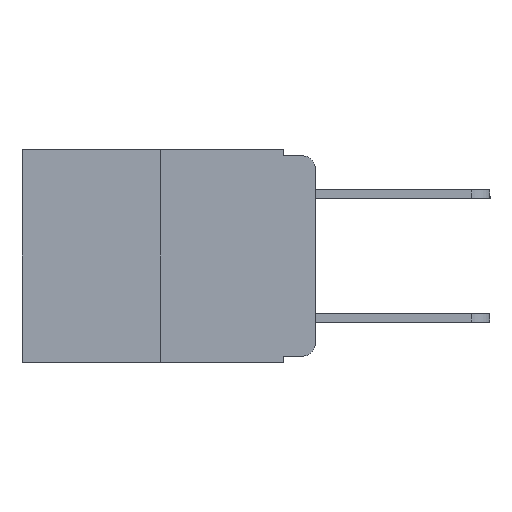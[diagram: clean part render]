
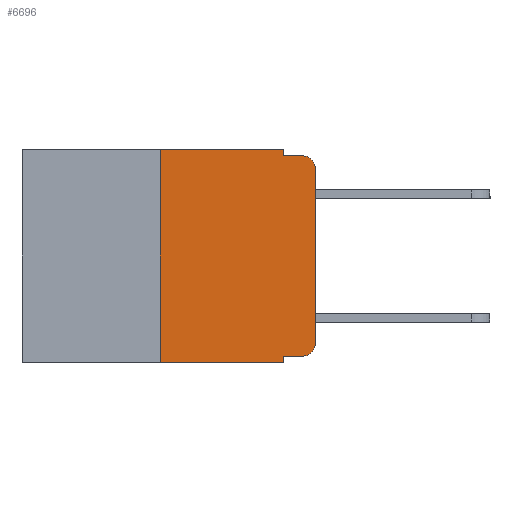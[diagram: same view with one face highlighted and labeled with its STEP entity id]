
A CAD part, left-side view. The second image highlights one B-rep face of the part: STEP entity #6696.
In plain terms, the highlighted planar face has unit normal (-1, 0, 0).
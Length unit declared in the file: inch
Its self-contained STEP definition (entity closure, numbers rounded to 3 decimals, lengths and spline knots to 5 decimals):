
#28 = LINE ( 'NONE', #1433, #3283 ) ;
#178 = CARTESIAN_POINT ( 'NONE',  ( 0., 0.051, -0.01 ) ) ;
#351 = DIRECTION ( 'NONE',  ( 0., 0., 1. ) ) ;
#733 = ORIENTED_EDGE ( 'NONE', *, *, #8186, .F. ) ;
#751 = ORIENTED_EDGE ( 'NONE', *, *, #13376, .T. ) ;
#1317 = VERTEX_POINT ( 'NONE', #10556 ) ;
#1433 = CARTESIAN_POINT ( 'NONE',  ( 0., 0.473, 0. ) ) ;
#1447 = DIRECTION ( 'NONE',  ( 0., -1., 0. ) ) ;
#2100 = ORIENTED_EDGE ( 'NONE', *, *, #13353, .T. ) ;
#2632 = DIRECTION ( 'NONE',  ( 0., -1., 0. ) ) ;
#3283 = VECTOR ( 'NONE', #2632, 39.37008 ) ;
#3311 = ORIENTED_EDGE ( 'NONE', *, *, #7199, .F. ) ;
#3335 = CARTESIAN_POINT ( 'NONE',  ( 0., 0.051, -0.333 ) ) ;
#3402 = ORIENTED_EDGE ( 'NONE', *, *, #8897, .T. ) ;
#3748 = FACE_OUTER_BOUND ( 'NONE', #5671, .T. ) ;
#3941 = VERTEX_POINT ( 'NONE', #10624 ) ;
#4159 = CARTESIAN_POINT ( 'NONE',  ( 0., 0., -0.313 ) ) ;
#4176 = DIRECTION ( 'NONE',  ( 0., 0., -1. ) ) ;
#4203 = LINE ( 'NONE', #178, #12463 ) ;
#4214 = CARTESIAN_POINT ( 'NONE',  ( 0., 0.25, 0. ) ) ;
#4242 = VECTOR ( 'NONE', #8245, 39.37008 ) ;
#4402 = VECTOR ( 'NONE', #13381, 39.37008 ) ;
#4470 = ORIENTED_EDGE ( 'NONE', *, *, #7860, .F. ) ;
#5124 = EDGE_CURVE ( 'NONE', #14193, #6923, #11903, .T. ) ;
#5505 = VERTEX_POINT ( 'NONE', #7129 ) ;
#5671 = EDGE_LOOP ( 'NONE', ( #13999, #6359, #7160, #733, #12368, #4470, #3402, #3311, #2100, #751 ) ) ;
#5741 = AXIS2_PLACEMENT_3D ( 'NONE', #7188, #6296, #4176 ) ;
#6055 = CARTESIAN_POINT ( 'NONE',  ( 0., 0.25, -0.343 ) ) ;
#6296 = DIRECTION ( 'NONE',  ( 1., 0., 0. ) ) ;
#6359 = ORIENTED_EDGE ( 'NONE', *, *, #5124, .T. ) ;
#6367 = CARTESIAN_POINT ( 'NONE',  ( 0., 0.051, 0. ) ) ;
#6696 = ADVANCED_FACE ( 'NONE', ( #3748 ), #10330, .F. ) ;
#6923 = VERTEX_POINT ( 'NONE', #14333 ) ;
#6975 = CARTESIAN_POINT ( 'NONE',  ( 0., 0.02, -0.313 ) ) ;
#7129 = CARTESIAN_POINT ( 'NONE',  ( 0., 0.051, -0.01 ) ) ;
#7160 = ORIENTED_EDGE ( 'NONE', *, *, #13539, .F. ) ;
#7188 = CARTESIAN_POINT ( 'NONE',  ( 0., 0.473, 0. ) ) ;
#7199 = EDGE_CURVE ( 'NONE', #3941, #11550, #14495, .T. ) ;
#7214 = CARTESIAN_POINT ( 'NONE',  ( 0., 0.051, 0. ) ) ;
#7386 = CARTESIAN_POINT ( 'NONE',  ( 0., 0.25, 0. ) ) ;
#7411 = CARTESIAN_POINT ( 'NONE',  ( 0., 0., -0.03 ) ) ;
#7500 = LINE ( 'NONE', #3335, #4402 ) ;
#7527 = DIRECTION ( 'NONE',  ( 0., 0., -1. ) ) ;
#7860 = EDGE_CURVE ( 'NONE', #11536, #13210, #8598, .T. ) ;
#8002 = DIRECTION ( 'NONE',  ( -1., 0., 0. ) ) ;
#8039 = VECTOR ( 'NONE', #12161, 39.37008 ) ;
#8068 = DIRECTION ( 'NONE',  ( 0., 0., -1. ) ) ;
#8104 = AXIS2_PLACEMENT_3D ( 'NONE', #6975, #14523, #8068 ) ;
#8186 = EDGE_CURVE ( 'NONE', #11513, #5505, #13182, .T. ) ;
#8245 = DIRECTION ( 'NONE',  ( 0., 0., -1. ) ) ;
#8556 = VECTOR ( 'NONE', #351, 39.37008 ) ;
#8598 = LINE ( 'NONE', #7386, #10826 ) ;
#8895 = LINE ( 'NONE', #13995, #8556 ) ;
#8897 = EDGE_CURVE ( 'NONE', #11536, #11550, #13810, .T. ) ;
#9282 = EDGE_CURVE ( 'NONE', #13210, #11513, #28, .T. ) ;
#10330 = PLANE ( 'NONE',  #5741 ) ;
#10508 = CARTESIAN_POINT ( 'NONE',  ( 0., 0.051, -0.343 ) ) ;
#10556 = CARTESIAN_POINT ( 'NONE',  ( 0., 0.02, -0.333 ) ) ;
#10624 = CARTESIAN_POINT ( 'NONE',  ( 0., 0.051, -0.333 ) ) ;
#10826 = VECTOR ( 'NONE', #13996, 39.37008 ) ;
#11072 = CARTESIAN_POINT ( 'NONE',  ( 0., 0.473, -0.343 ) ) ;
#11164 = VERTEX_POINT ( 'NONE', #4159 ) ;
#11450 = CARTESIAN_POINT ( 'NONE',  ( 0., 0.051, 0. ) ) ;
#11513 = VERTEX_POINT ( 'NONE', #11450 ) ;
#11536 = VERTEX_POINT ( 'NONE', #6055 ) ;
#11550 = VERTEX_POINT ( 'NONE', #10508 ) ;
#11587 = AXIS2_PLACEMENT_3D ( 'NONE', #12296, #8002, #7527 ) ;
#11667 = VECTOR ( 'NONE', #12500, 39.37008 ) ;
#11903 = CIRCLE ( 'NONE', #11587, 0.02 ) ;
#12161 = DIRECTION ( 'NONE',  ( 0., -1., 0. ) ) ;
#12296 = CARTESIAN_POINT ( 'NONE',  ( 0., 0.02, -0.03 ) ) ;
#12368 = ORIENTED_EDGE ( 'NONE', *, *, #9282, .F. ) ;
#12463 = VECTOR ( 'NONE', #1447, 39.37008 ) ;
#12500 = DIRECTION ( 'NONE',  ( 0., 0., -1. ) ) ;
#12980 = CIRCLE ( 'NONE', #8104, 0.02 ) ;
#13182 = LINE ( 'NONE', #7214, #4242 ) ;
#13210 = VERTEX_POINT ( 'NONE', #4214 ) ;
#13353 = EDGE_CURVE ( 'NONE', #3941, #1317, #7500, .T. ) ;
#13376 = EDGE_CURVE ( 'NONE', #1317, #11164, #12980, .T. ) ;
#13381 = DIRECTION ( 'NONE',  ( 0., -1., 0. ) ) ;
#13539 = EDGE_CURVE ( 'NONE', #5505, #6923, #4203, .T. ) ;
#13640 = EDGE_CURVE ( 'NONE', #11164, #14193, #8895, .T. ) ;
#13810 = LINE ( 'NONE', #11072, #8039 ) ;
#13995 = CARTESIAN_POINT ( 'NONE',  ( 0., 0., 0. ) ) ;
#13996 = DIRECTION ( 'NONE',  ( 0., 0., 1. ) ) ;
#13999 = ORIENTED_EDGE ( 'NONE', *, *, #13640, .T. ) ;
#14193 = VERTEX_POINT ( 'NONE', #7411 ) ;
#14333 = CARTESIAN_POINT ( 'NONE',  ( 0., 0.02, -0.01 ) ) ;
#14495 = LINE ( 'NONE', #6367, #11667 ) ;
#14523 = DIRECTION ( 'NONE',  ( -1., 0., 0. ) ) ;
